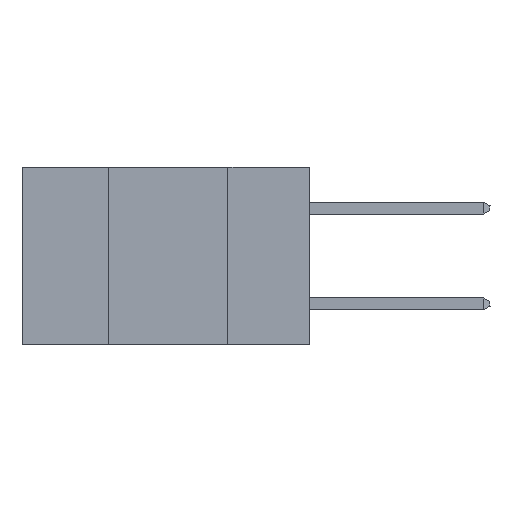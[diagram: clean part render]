
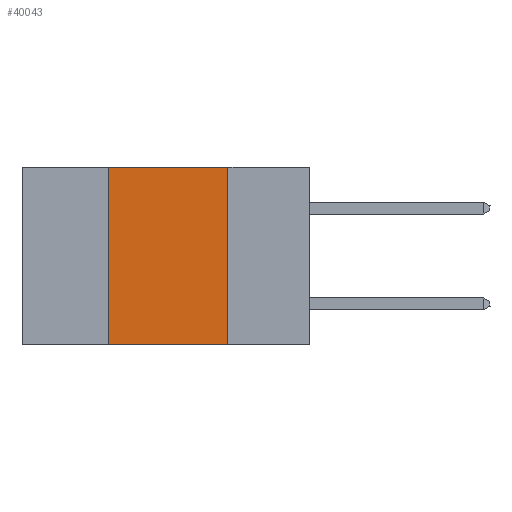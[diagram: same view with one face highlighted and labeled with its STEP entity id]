
A CAD part, left-side view. The second image highlights one B-rep face of the part: STEP entity #40043.
In plain terms, the highlighted planar face has unit normal (-1, 0, 0).
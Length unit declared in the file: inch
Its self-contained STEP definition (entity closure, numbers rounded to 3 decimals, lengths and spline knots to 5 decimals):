
#615 = CARTESIAN_POINT ( 'NONE',  ( 0., 0.6, 0. ) ) ;
#2642 = EDGE_CURVE ( 'NONE', #9634, #40134, #5794, .T. ) ;
#3446 = DIRECTION ( 'NONE',  ( 0., 0., -1. ) ) ;
#3599 = ORIENTED_EDGE ( 'NONE', *, *, #21290, .F. ) ;
#4754 = CARTESIAN_POINT ( 'NONE',  ( 0., 0.17, 0. ) ) ;
#5794 = LINE ( 'NONE', #9913, #30865 ) ;
#6885 = LINE ( 'NONE', #24360, #38413 ) ;
#7327 = ORIENTED_EDGE ( 'NONE', *, *, #2642, .F. ) ;
#8185 = ORIENTED_EDGE ( 'NONE', *, *, #26486, .T. ) ;
#9634 = VERTEX_POINT ( 'NONE', #26216 ) ;
#9913 = CARTESIAN_POINT ( 'NONE',  ( 0., 0.6, 0. ) ) ;
#11286 = VECTOR ( 'NONE', #24090, 39.37008 ) ;
#12059 = DIRECTION ( 'NONE',  ( 0., 0., 1. ) ) ;
#13527 = LINE ( 'NONE', #23977, #19050 ) ;
#14079 = CARTESIAN_POINT ( 'NONE',  ( 0., 0.17, 0. ) ) ;
#16254 = VERTEX_POINT ( 'NONE', #22089 ) ;
#19050 = VECTOR ( 'NONE', #36510, 39.37008 ) ;
#19741 = DIRECTION ( 'NONE',  ( 0., -1., 0. ) ) ;
#19945 = VERTEX_POINT ( 'NONE', #30137 ) ;
#21290 = EDGE_CURVE ( 'NONE', #16254, #9634, #6885, .T. ) ;
#22089 = CARTESIAN_POINT ( 'NONE',  ( 0., 0.42, -0.37 ) ) ;
#22752 = PLANE ( 'NONE',  #34791 ) ;
#23874 = ORIENTED_EDGE ( 'NONE', *, *, #35504, .F. ) ;
#23977 = CARTESIAN_POINT ( 'NONE',  ( 0., 0.6, -0.37 ) ) ;
#24090 = DIRECTION ( 'NONE',  ( 0., 0., -1. ) ) ;
#24360 = CARTESIAN_POINT ( 'NONE',  ( 0., 0.42, 0. ) ) ;
#26216 = CARTESIAN_POINT ( 'NONE',  ( 0., 0.42, 0. ) ) ;
#26376 = EDGE_LOOP ( 'NONE', ( #23874, #7327, #3599, #8185 ) ) ;
#26486 = EDGE_CURVE ( 'NONE', #16254, #19945, #13527, .T. ) ;
#30137 = CARTESIAN_POINT ( 'NONE',  ( 0., 0.17, -0.37 ) ) ;
#30865 = VECTOR ( 'NONE', #19741, 39.37008 ) ;
#32365 = FACE_OUTER_BOUND ( 'NONE', #26376, .T. ) ;
#32804 = DIRECTION ( 'NONE',  ( 1., 0., 0. ) ) ;
#34791 = AXIS2_PLACEMENT_3D ( 'NONE', #615, #32804, #3446 ) ;
#35504 = EDGE_CURVE ( 'NONE', #40134, #19945, #38754, .T. ) ;
#36510 = DIRECTION ( 'NONE',  ( 0., -1., 0. ) ) ;
#38413 = VECTOR ( 'NONE', #12059, 39.37008 ) ;
#38754 = LINE ( 'NONE', #4754, #11286 ) ;
#40043 = ADVANCED_FACE ( 'NONE', ( #32365 ), #22752, .F. ) ;
#40134 = VERTEX_POINT ( 'NONE', #14079 ) ;
